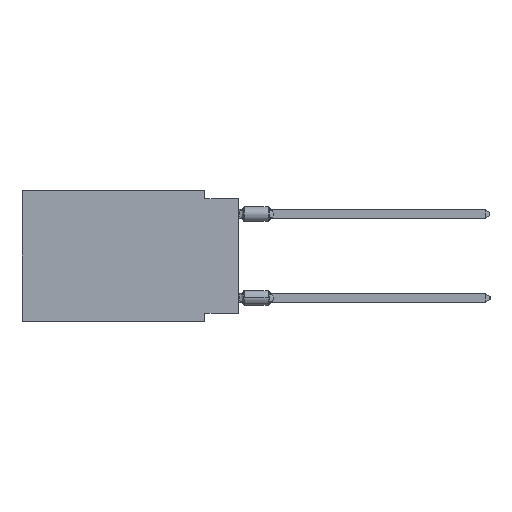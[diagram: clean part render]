
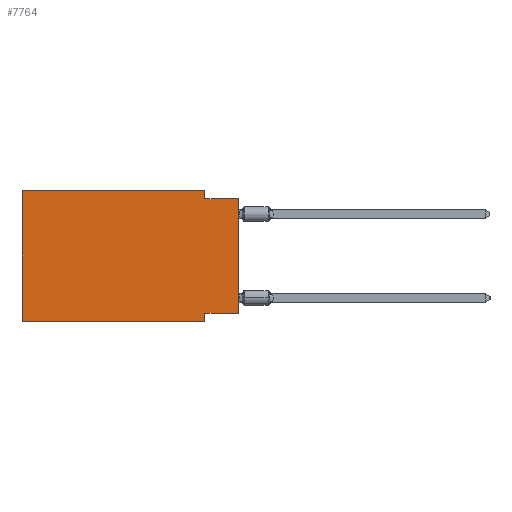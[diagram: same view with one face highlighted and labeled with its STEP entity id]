
A CAD part, left-side view. The second image highlights one B-rep face of the part: STEP entity #7764.
In plain terms, the highlighted planar face has unit normal (-1, 0, 0).
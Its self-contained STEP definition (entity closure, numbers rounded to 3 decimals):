
#42 = VERTEX_POINT ( 'NONE', #36027 ) ;
#1130 = DIRECTION ( 'NONE',  ( 0., 0., 1. ) ) ;
#2589 = DIRECTION ( 'NONE',  ( 0., 0., 1. ) ) ;
#2612 = DIRECTION ( 'NONE',  ( 1., 0., 0. ) ) ;
#4233 = VERTEX_POINT ( 'NONE', #28781 ) ;
#6753 = CARTESIAN_POINT ( 'NONE',  ( 0., 0., -0.635 ) ) ;
#6767 = DIRECTION ( 'NONE',  ( 0., -1., 0. ) ) ;
#7357 = ORIENTED_EDGE ( 'NONE', *, *, #23237, .F. ) ;
#7764 = ADVANCED_FACE ( 'NONE', ( #19928 ), #33418, .F. ) ;
#7873 = CARTESIAN_POINT ( 'NONE',  ( 0., 2.54, -9.271 ) ) ;
#8374 = ORIENTED_EDGE ( 'NONE', *, *, #27892, .F. ) ;
#9293 = LINE ( 'NONE', #32753, #12214 ) ;
#10261 = DIRECTION ( 'NONE',  ( 0., 1., 0. ) ) ;
#10456 = LINE ( 'NONE', #23982, #16303 ) ;
#11053 = VERTEX_POINT ( 'NONE', #18287 ) ;
#12214 = VECTOR ( 'NONE', #16387, 1000. ) ;
#13421 = CARTESIAN_POINT ( 'NONE',  ( 0., 0., -9.271 ) ) ;
#13799 = CARTESIAN_POINT ( 'NONE',  ( 0., 0., -9.271 ) ) ;
#13967 = EDGE_LOOP ( 'NONE', ( #34491, #27660, #14242, #8374, #7357, #15761, #43576, #14657 ) ) ;
#14242 = ORIENTED_EDGE ( 'NONE', *, *, #35591, .F. ) ;
#14657 = ORIENTED_EDGE ( 'NONE', *, *, #42758, .F. ) ;
#14942 = EDGE_CURVE ( 'NONE', #19558, #11053, #10456, .T. ) ;
#15419 = VECTOR ( 'NONE', #39278, 1000. ) ;
#15635 = AXIS2_PLACEMENT_3D ( 'NONE', #32965, #2612, #29441 ) ;
#15761 = ORIENTED_EDGE ( 'NONE', *, *, #14942, .T. ) ;
#16303 = VECTOR ( 'NONE', #37695, 1000. ) ;
#16313 = LINE ( 'NONE', #19855, #32782 ) ;
#16387 = DIRECTION ( 'NONE',  ( 0., 0., -1. ) ) ;
#17564 = CARTESIAN_POINT ( 'NONE',  ( 0., 16.383, 0. ) ) ;
#17603 = VECTOR ( 'NONE', #2589, 1000. ) ;
#18287 = CARTESIAN_POINT ( 'NONE',  ( 0., 2.54, -9.906 ) ) ;
#19153 = CARTESIAN_POINT ( 'NONE',  ( 0., 2.54, 0. ) ) ;
#19558 = VERTEX_POINT ( 'NONE', #41433 ) ;
#19855 = CARTESIAN_POINT ( 'NONE',  ( 0., 16.383, 0. ) ) ;
#19928 = FACE_OUTER_BOUND ( 'NONE', #13967, .T. ) ;
#20486 = LINE ( 'NONE', #6753, #23551 ) ;
#20873 = EDGE_CURVE ( 'NONE', #42, #26515, #20486, .T. ) ;
#21132 = DIRECTION ( 'NONE',  ( 0., -1., 0. ) ) ;
#21529 = EDGE_CURVE ( 'NONE', #29106, #26515, #33811, .T. ) ;
#23237 = EDGE_CURVE ( 'NONE', #19558, #38226, #24875, .T. ) ;
#23551 = VECTOR ( 'NONE', #21132, 1000. ) ;
#23982 = CARTESIAN_POINT ( 'NONE',  ( 0., 16.383, -9.906 ) ) ;
#24875 = LINE ( 'NONE', #17564, #38892 ) ;
#26515 = VERTEX_POINT ( 'NONE', #34726 ) ;
#27660 = ORIENTED_EDGE ( 'NONE', *, *, #20873, .F. ) ;
#27892 = EDGE_CURVE ( 'NONE', #38226, #4233, #16313, .T. ) ;
#28228 = VECTOR ( 'NONE', #10261, 1000. ) ;
#28551 = EDGE_CURVE ( 'NONE', #29183, #11053, #9293, .T. ) ;
#28781 = CARTESIAN_POINT ( 'NONE',  ( 0., 2.54, 0. ) ) ;
#29106 = VERTEX_POINT ( 'NONE', #13421 ) ;
#29183 = VERTEX_POINT ( 'NONE', #7873 ) ;
#29441 = DIRECTION ( 'NONE',  ( 0., 0., -1. ) ) ;
#30425 = LINE ( 'NONE', #13799, #28228 ) ;
#32753 = CARTESIAN_POINT ( 'NONE',  ( 0., 2.54, -9.906 ) ) ;
#32782 = VECTOR ( 'NONE', #6767, 1000. ) ;
#32965 = CARTESIAN_POINT ( 'NONE',  ( 0., 16.383, 0. ) ) ;
#33418 = PLANE ( 'NONE',  #15635 ) ;
#33811 = LINE ( 'NONE', #36479, #17603 ) ;
#34491 = ORIENTED_EDGE ( 'NONE', *, *, #21529, .T. ) ;
#34726 = CARTESIAN_POINT ( 'NONE',  ( 0., 0., -0.635 ) ) ;
#35591 = EDGE_CURVE ( 'NONE', #4233, #42, #42616, .T. ) ;
#36027 = CARTESIAN_POINT ( 'NONE',  ( 0., 2.54, -0.635 ) ) ;
#36479 = CARTESIAN_POINT ( 'NONE',  ( 0., 0., 0. ) ) ;
#37695 = DIRECTION ( 'NONE',  ( 0., -1., 0. ) ) ;
#38226 = VERTEX_POINT ( 'NONE', #42464 ) ;
#38892 = VECTOR ( 'NONE', #1130, 1000. ) ;
#39278 = DIRECTION ( 'NONE',  ( 0., 0., -1. ) ) ;
#41433 = CARTESIAN_POINT ( 'NONE',  ( 0., 16.383, -9.906 ) ) ;
#42464 = CARTESIAN_POINT ( 'NONE',  ( 0., 16.383, 0. ) ) ;
#42616 = LINE ( 'NONE', #19153, #15419 ) ;
#42758 = EDGE_CURVE ( 'NONE', #29106, #29183, #30425, .T. ) ;
#43576 = ORIENTED_EDGE ( 'NONE', *, *, #28551, .F. ) ;
